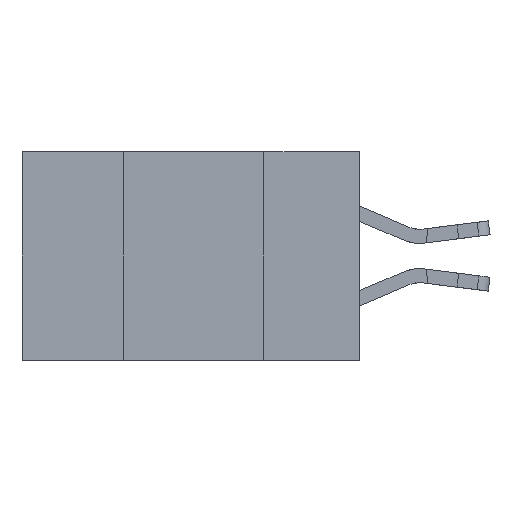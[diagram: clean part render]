
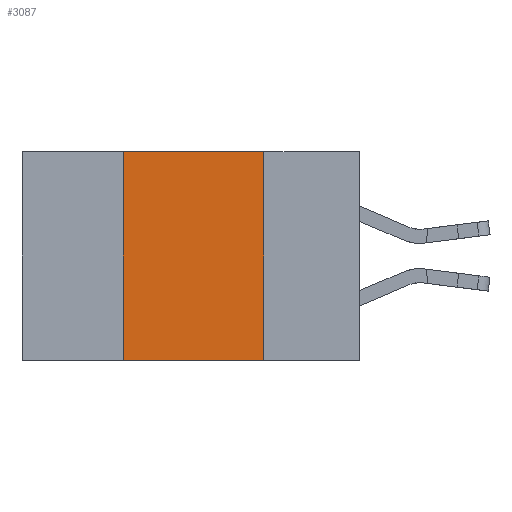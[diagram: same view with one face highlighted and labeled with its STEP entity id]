
A CAD part, left-side view. The second image highlights one B-rep face of the part: STEP entity #3087.
In plain terms, the highlighted planar face has unit normal (-1, 0, 0).
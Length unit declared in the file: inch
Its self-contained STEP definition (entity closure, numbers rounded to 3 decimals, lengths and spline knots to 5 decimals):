
#1001 = CARTESIAN_POINT ( 'NONE',  ( 0., 0.42, 0. ) ) ;
#3001 = VERTEX_POINT ( 'NONE', #3981 ) ;
#3087 = ADVANCED_FACE ( 'NONE', ( #4557 ), #8645, .F. ) ;
#3981 = CARTESIAN_POINT ( 'NONE',  ( 0., 0.17, 0. ) ) ;
#4062 = CARTESIAN_POINT ( 'NONE',  ( 0., 0.6, 0. ) ) ;
#4557 = FACE_OUTER_BOUND ( 'NONE', #23489, .T. ) ;
#5068 = DIRECTION ( 'NONE',  ( 0., 0., 1. ) ) ;
#5896 = LINE ( 'NONE', #4062, #15266 ) ;
#5960 = VERTEX_POINT ( 'NONE', #1001 ) ;
#7443 = EDGE_CURVE ( 'NONE', #3001, #19170, #11891, .T. ) ;
#8318 = VECTOR ( 'NONE', #20261, 39.37008 ) ;
#8389 = ORIENTED_EDGE ( 'NONE', *, *, #7443, .F. ) ;
#8645 = PLANE ( 'NONE',  #18944 ) ;
#8932 = LINE ( 'NONE', #15984, #15957 ) ;
#9766 = LINE ( 'NONE', #9894, #13587 ) ;
#9894 = CARTESIAN_POINT ( 'NONE',  ( 0., 0.6, -0.37 ) ) ;
#10470 = ORIENTED_EDGE ( 'NONE', *, *, #13160, .T. ) ;
#10491 = DIRECTION ( 'NONE',  ( 1., 0., 0. ) ) ;
#11371 = CARTESIAN_POINT ( 'NONE',  ( 0., 0.17, -0.37 ) ) ;
#11790 = DIRECTION ( 'NONE',  ( 0., -1., 0. ) ) ;
#11891 = LINE ( 'NONE', #12789, #8318 ) ;
#12315 = CARTESIAN_POINT ( 'NONE',  ( 0., 0.6, 0. ) ) ;
#12789 = CARTESIAN_POINT ( 'NONE',  ( 0., 0.17, 0. ) ) ;
#13089 = CARTESIAN_POINT ( 'NONE',  ( 0., 0.42, -0.37 ) ) ;
#13160 = EDGE_CURVE ( 'NONE', #19038, #19170, #9766, .T. ) ;
#13587 = VECTOR ( 'NONE', #11790, 39.37008 ) ;
#15266 = VECTOR ( 'NONE', #21098, 39.37008 ) ;
#15957 = VECTOR ( 'NONE', #5068, 39.37008 ) ;
#15984 = CARTESIAN_POINT ( 'NONE',  ( 0., 0.42, 0. ) ) ;
#16452 = ORIENTED_EDGE ( 'NONE', *, *, #22520, .F. ) ;
#17858 = EDGE_CURVE ( 'NONE', #5960, #3001, #5896, .T. ) ;
#18944 = AXIS2_PLACEMENT_3D ( 'NONE', #12315, #10491, #23551 ) ;
#19038 = VERTEX_POINT ( 'NONE', #13089 ) ;
#19170 = VERTEX_POINT ( 'NONE', #11371 ) ;
#20261 = DIRECTION ( 'NONE',  ( 0., 0., -1. ) ) ;
#21098 = DIRECTION ( 'NONE',  ( 0., -1., 0. ) ) ;
#22306 = ORIENTED_EDGE ( 'NONE', *, *, #17858, .F. ) ;
#22520 = EDGE_CURVE ( 'NONE', #19038, #5960, #8932, .T. ) ;
#23489 = EDGE_LOOP ( 'NONE', ( #8389, #22306, #16452, #10470 ) ) ;
#23551 = DIRECTION ( 'NONE',  ( 0., 0., -1. ) ) ;
